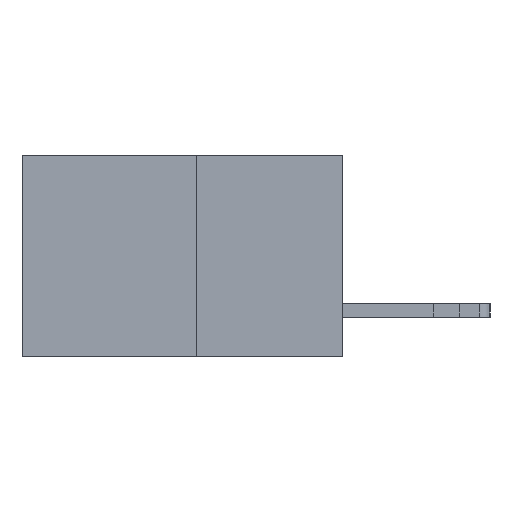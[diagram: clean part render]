
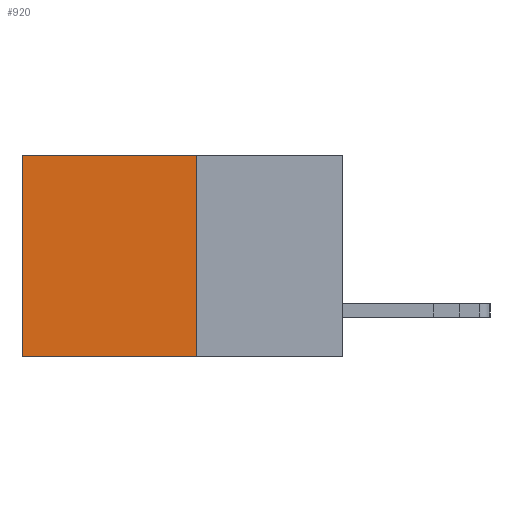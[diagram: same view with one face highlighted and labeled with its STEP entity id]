
A CAD part, left-side view. The second image highlights one B-rep face of the part: STEP entity #920.
In plain terms, the highlighted planar face has unit normal (-1, 0, 0).
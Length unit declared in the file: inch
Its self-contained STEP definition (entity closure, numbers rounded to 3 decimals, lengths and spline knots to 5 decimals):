
#270 = ORIENTED_EDGE ( 'NONE', *, *, #1585, .F. ) ;
#342 = LINE ( 'NONE', #1212, #12967 ) ;
#436 = LINE ( 'NONE', #7887, #3016 ) ;
#868 = CARTESIAN_POINT ( 'NONE',  ( 0.277, 0.27, 0. ) ) ;
#920 = ADVANCED_FACE ( 'NONE', ( #14804 ), #4597, .F. ) ;
#1212 = CARTESIAN_POINT ( 'NONE',  ( 0.277, 0.27, -0.37 ) ) ;
#1457 = EDGE_LOOP ( 'NONE', ( #2690, #270, #3092, #10732 ) ) ;
#1585 = EDGE_CURVE ( 'NONE', #6792, #2992, #12148, .T. ) ;
#2507 = CARTESIAN_POINT ( 'NONE',  ( 0.277, 0.27, -0.37 ) ) ;
#2690 = ORIENTED_EDGE ( 'NONE', *, *, #4208, .T. ) ;
#2992 = VERTEX_POINT ( 'NONE', #15056 ) ;
#3016 = VECTOR ( 'NONE', #7588, 39.37008 ) ;
#3072 = VECTOR ( 'NONE', #7106, 39.37008 ) ;
#3092 = ORIENTED_EDGE ( 'NONE', *, *, #6739, .F. ) ;
#3470 = LINE ( 'NONE', #868, #3072 ) ;
#4208 = EDGE_CURVE ( 'NONE', #6642, #2992, #436, .T. ) ;
#4597 = PLANE ( 'NONE',  #8165 ) ;
#6412 = DIRECTION ( 'NONE',  ( 0., 0., -1. ) ) ;
#6461 = CARTESIAN_POINT ( 'NONE',  ( 0.277, 0.59, 0. ) ) ;
#6509 = VERTEX_POINT ( 'NONE', #6799 ) ;
#6642 = VERTEX_POINT ( 'NONE', #6461 ) ;
#6739 = EDGE_CURVE ( 'NONE', #6509, #6792, #342, .T. ) ;
#6792 = VERTEX_POINT ( 'NONE', #2507 ) ;
#6799 = CARTESIAN_POINT ( 'NONE',  ( 0.277, 0.27, 0. ) ) ;
#7106 = DIRECTION ( 'NONE',  ( 0., 1., 0. ) ) ;
#7588 = DIRECTION ( 'NONE',  ( 0., 0., -1. ) ) ;
#7887 = CARTESIAN_POINT ( 'NONE',  ( 0.277, 0.59, -0.37 ) ) ;
#8165 = AXIS2_PLACEMENT_3D ( 'NONE', #10699, #12797, #14808 ) ;
#8967 = VECTOR ( 'NONE', #11415, 39.37008 ) ;
#9494 = CARTESIAN_POINT ( 'NONE',  ( 0.277, 0.27, -0.37 ) ) ;
#9525 = EDGE_CURVE ( 'NONE', #6509, #6642, #3470, .T. ) ;
#10699 = CARTESIAN_POINT ( 'NONE',  ( 0.277, 0.27, -0.37 ) ) ;
#10732 = ORIENTED_EDGE ( 'NONE', *, *, #9525, .T. ) ;
#11415 = DIRECTION ( 'NONE',  ( 0., 1., 0. ) ) ;
#12148 = LINE ( 'NONE', #9494, #8967 ) ;
#12797 = DIRECTION ( 'NONE',  ( 1., 0., 0. ) ) ;
#12967 = VECTOR ( 'NONE', #6412, 39.37008 ) ;
#14804 = FACE_OUTER_BOUND ( 'NONE', #1457, .T. ) ;
#14808 = DIRECTION ( 'NONE',  ( 0., 0., -1. ) ) ;
#15056 = CARTESIAN_POINT ( 'NONE',  ( 0.277, 0.59, -0.37 ) ) ;
